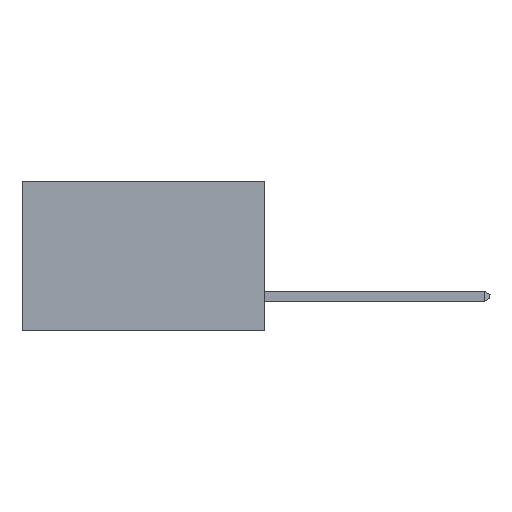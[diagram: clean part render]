
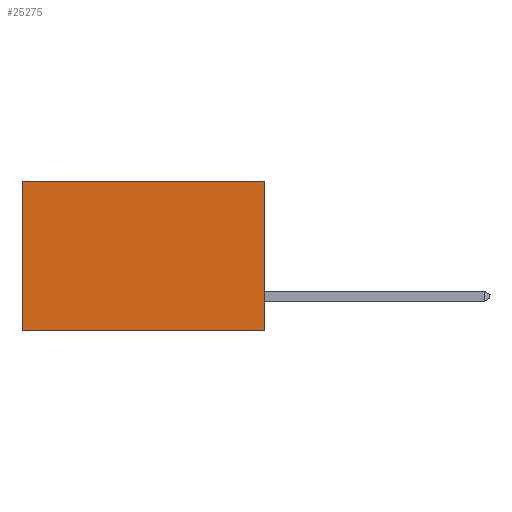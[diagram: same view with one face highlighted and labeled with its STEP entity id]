
A CAD part, left-side view. The second image highlights one B-rep face of the part: STEP entity #25275.
In plain terms, the highlighted planar face has unit normal (-1, 0, 0).
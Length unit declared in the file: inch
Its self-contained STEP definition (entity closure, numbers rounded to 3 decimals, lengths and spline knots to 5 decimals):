
#249 = VERTEX_POINT ( 'NONE', #5381 ) ;
#641 = AXIS2_PLACEMENT_3D ( 'NONE', #6938, #10929, #8845 ) ;
#1643 = EDGE_CURVE ( 'NONE', #16112, #21061, #7971, .T. ) ;
#1969 = ORIENTED_EDGE ( 'NONE', *, *, #3478, .T. ) ;
#2574 = FACE_OUTER_BOUND ( 'NONE', #15345, .T. ) ;
#3478 = EDGE_CURVE ( 'NONE', #16112, #249, #6339, .T. ) ;
#4318 = CARTESIAN_POINT ( 'NONE',  ( 0.298, 0.6, 0. ) ) ;
#4954 = DIRECTION ( 'NONE',  ( 0., 1., 0. ) ) ;
#5106 = ORIENTED_EDGE ( 'NONE', *, *, #11729, .F. ) ;
#5381 = CARTESIAN_POINT ( 'NONE',  ( 0.298, 0.6, 0. ) ) ;
#6339 = LINE ( 'NONE', #9228, #23566 ) ;
#6938 = CARTESIAN_POINT ( 'NONE',  ( 0.298, 0., 0. ) ) ;
#7685 = VECTOR ( 'NONE', #23870, 39.37008 ) ;
#7971 = LINE ( 'NONE', #24109, #16606 ) ;
#8169 = CARTESIAN_POINT ( 'NONE',  ( 0.298, 0.6, -0.37 ) ) ;
#8845 = DIRECTION ( 'NONE',  ( 0., 0., -1. ) ) ;
#9228 = CARTESIAN_POINT ( 'NONE',  ( 0.298, 0., 0. ) ) ;
#10146 = ORIENTED_EDGE ( 'NONE', *, *, #1643, .F. ) ;
#10609 = CARTESIAN_POINT ( 'NONE',  ( 0.298, 0., -0.37 ) ) ;
#10929 = DIRECTION ( 'NONE',  ( 1., 0., 0. ) ) ;
#11729 = EDGE_CURVE ( 'NONE', #21061, #19347, #21518, .T. ) ;
#12319 = LINE ( 'NONE', #4318, #7685 ) ;
#12353 = DIRECTION ( 'NONE',  ( 0., 0., -1. ) ) ;
#15345 = EDGE_LOOP ( 'NONE', ( #20932, #5106, #10146, #1969 ) ) ;
#16112 = VERTEX_POINT ( 'NONE', #21429 ) ;
#16606 = VECTOR ( 'NONE', #12353, 39.37008 ) ;
#19347 = VERTEX_POINT ( 'NONE', #8169 ) ;
#19880 = CARTESIAN_POINT ( 'NONE',  ( 0.298, 0., -0.37 ) ) ;
#20447 = PLANE ( 'NONE',  #641 ) ;
#20909 = DIRECTION ( 'NONE',  ( 0., 1., 0. ) ) ;
#20932 = ORIENTED_EDGE ( 'NONE', *, *, #21114, .T. ) ;
#21061 = VERTEX_POINT ( 'NONE', #19880 ) ;
#21114 = EDGE_CURVE ( 'NONE', #249, #19347, #12319, .T. ) ;
#21429 = CARTESIAN_POINT ( 'NONE',  ( 0.298, 0., 0. ) ) ;
#21518 = LINE ( 'NONE', #10609, #22748 ) ;
#22748 = VECTOR ( 'NONE', #4954, 39.37008 ) ;
#23566 = VECTOR ( 'NONE', #20909, 39.37008 ) ;
#23870 = DIRECTION ( 'NONE',  ( 0., 0., -1. ) ) ;
#24109 = CARTESIAN_POINT ( 'NONE',  ( 0.298, 0., 0. ) ) ;
#25275 = ADVANCED_FACE ( 'NONE', ( #2574 ), #20447, .F. ) ;
